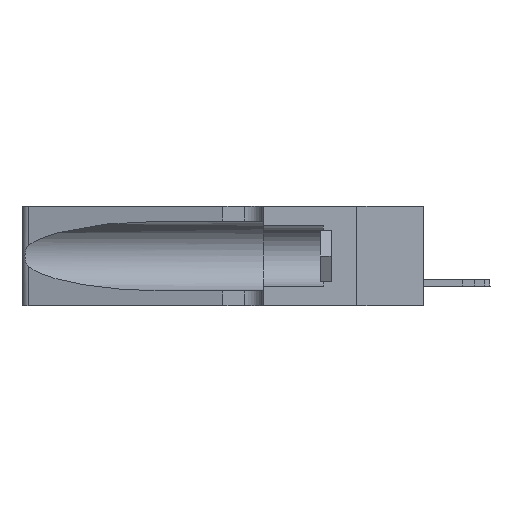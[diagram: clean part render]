
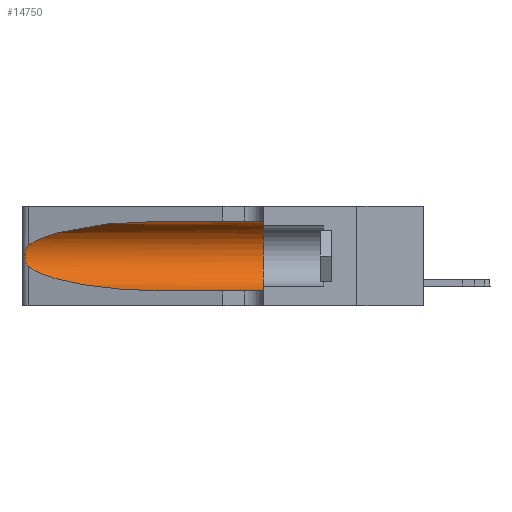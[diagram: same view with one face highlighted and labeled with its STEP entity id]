
A CAD part, left-side view. The second image highlights one B-rep face of the part: STEP entity #14750.
In plain terms, the highlighted cylindrical face has radius 3.308 mm (diameter 6.617 mm), a partial arc.
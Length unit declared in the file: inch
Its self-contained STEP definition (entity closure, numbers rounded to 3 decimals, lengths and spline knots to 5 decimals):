
#248 = CARTESIAN_POINT ( 'NONE',  ( 0.25854, 1.2359, 0.20912 ) ) ;
#848 = CARTESIAN_POINT ( 'NONE',  ( 0.25487, 1.22718, 0.14631 ) ) ;
#2346 = AXIS2_PLACEMENT_3D ( 'NONE', #15928, #9743, #16616 ) ;
#2508 = CARTESIAN_POINT ( 'NONE',  ( 0.1305, 0.35, 0.05475 ) ) ;
#2638 = DIRECTION ( 'NONE',  ( 0., 0., 1. ) ) ;
#3244 = VERTEX_POINT ( 'NONE', #22983 ) ;
#3895 = VERTEX_POINT ( 'NONE', #26742 ) ;
#4047 = EDGE_CURVE ( 'NONE', #18157, #18648, #27140, .T. ) ;
#4755 = ORIENTED_EDGE ( 'NONE', *, *, #14588, .T. ) ;
#4892 = CARTESIAN_POINT ( 'NONE',  ( 0.25487, 1.22718, 0.14631 ) ) ;
#5075 = CARTESIAN_POINT ( 'NONE',  ( 0.26075, 1.23896, 0.19203 ) ) ;
#5078 = DIRECTION ( 'NONE',  ( 0., -1., 0. ) ) ;
#5647 = VECTOR ( 'NONE', #5078, 39.37008 ) ;
#6132 = CARTESIAN_POINT ( 'NONE',  ( 0.25487, 1.22718, 0.22369 ) ) ;
#6234 = CARTESIAN_POINT ( 'NONE',  ( 0.25555, 1.22994, 0.2215 ) ) ;
#7052 = CARTESIAN_POINT ( 'NONE',  ( 0.1305, 0.72297, 0.31525 ) ) ;
#7231 = CARTESIAN_POINT ( 'NONE',  ( 0.26018, 1.23835, 0.19895 ) ) ;
#7365 = ORIENTED_EDGE ( 'NONE', *, *, #4047, .F. ) ;
#7531 = CARTESIAN_POINT ( 'NONE',  ( 0.25856, 1.23593, 0.16098 ) ) ;
#7639 = EDGE_CURVE ( 'NONE', #11296, #3895, #25047, .T. ) ;
#7738 = EDGE_CURVE ( 'NONE', #3895, #3244, #27250, .T. ) ;
#7966 = CYLINDRICAL_SURFACE ( 'NONE', #2346, 0.13025 ) ;
#8201 = CARTESIAN_POINT ( 'NONE',  ( 0.1305, 1.61858, 0.05475 ) ) ;
#8306 = DIRECTION ( 'NONE',  ( 0., -1., 0. ) ) ;
#9164 = LINE ( 'NONE', #11592, #5647 ) ;
#9306 = CARTESIAN_POINT ( 'NONE',  ( 0.18966, 0.96281, 0.31525 ) ) ;
#9743 = DIRECTION ( 'NONE',  ( 0., -1., 0. ) ) ;
#10112 =( BOUNDED_CURVE ( )  B_SPLINE_CURVE ( 3, ( #4892, #11691, #27488, #16175 ),
 .UNSPECIFIED., .F., .F. ) 
 B_SPLINE_CURVE_WITH_KNOTS ( ( 4, 4 ),
 ( 3.44316, 4.71239 ),
 .UNSPECIFIED. ) 
 CURVE ( )  GEOMETRIC_REPRESENTATION_ITEM ( )  RATIONAL_B_SPLINE_CURVE ( ( 1., 0.87, 0.87, 1. ) ) 
 REPRESENTATION_ITEM ( '' )  );
#11251 = EDGE_LOOP ( 'NONE', ( #20474, #21062, #4755, #28572, #7365, #18052 ) ) ;
#11296 = VERTEX_POINT ( 'NONE', #13615 ) ;
#11592 = CARTESIAN_POINT ( 'NONE',  ( 0.1305, 1.61858, 0.31525 ) ) ;
#11691 = CARTESIAN_POINT ( 'NONE',  ( 0.2373, 1.15595, 0.08982 ) ) ;
#12273 = CARTESIAN_POINT ( 'NONE',  ( 0.25639, 1.23186, 0.15144 ) ) ;
#13034 = EDGE_CURVE ( 'NONE', #16992, #18648, #18766, .T. ) ;
#13615 = CARTESIAN_POINT ( 'NONE',  ( 0.1305, 0.72297, 0.31525 ) ) ;
#13805 = CARTESIAN_POINT ( 'NONE',  ( 0.26075, 1.23896, 0.178 ) ) ;
#13905 = CARTESIAN_POINT ( 'NONE',  ( 0.26017, 1.23833, 0.17102 ) ) ;
#14387 = CARTESIAN_POINT ( 'NONE',  ( 0.1305, 0.72297, 0.05475 ) ) ;
#14588 = EDGE_CURVE ( 'NONE', #3244, #16992, #10112, .T. ) ;
#14750 = ADVANCED_FACE ( 'NONE', ( #16508 ), #7966, .F. ) ;
#15928 = CARTESIAN_POINT ( 'NONE',  ( 0.1305, 1.61858, 0.185 ) ) ;
#16175 = CARTESIAN_POINT ( 'NONE',  ( 0.1305, 0.72297, 0.05475 ) ) ;
#16508 = FACE_OUTER_BOUND ( 'NONE', #11251, .T. ) ;
#16616 = DIRECTION ( 'NONE',  ( 0., 0., -1. ) ) ;
#16992 = VERTEX_POINT ( 'NONE', #14387 ) ;
#18052 = ORIENTED_EDGE ( 'NONE', *, *, #28957, .F. ) ;
#18157 = VERTEX_POINT ( 'NONE', #25216 ) ;
#18260 = CARTESIAN_POINT ( 'NONE',  ( 0.25787, 1.23484, 0.2124 ) ) ;
#18648 = VERTEX_POINT ( 'NONE', #2508 ) ;
#18766 = LINE ( 'NONE', #8201, #25119 ) ;
#20474 = ORIENTED_EDGE ( 'NONE', *, *, #7639, .T. ) ;
#20752 = CARTESIAN_POINT ( 'NONE',  ( 0.25487, 1.22718, 0.22369 ) ) ;
#20764 = CARTESIAN_POINT ( 'NONE',  ( 0.1305, 0.35, 0.185 ) ) ;
#20847 = CARTESIAN_POINT ( 'NONE',  ( 0.25639, 1.23184, 0.21858 ) ) ;
#21062 = ORIENTED_EDGE ( 'NONE', *, *, #7738, .T. ) ;
#22983 = CARTESIAN_POINT ( 'NONE',  ( 0.25487, 1.22718, 0.14631 ) ) ;
#23315 = CARTESIAN_POINT ( 'NONE',  ( 0.25555, 1.22993, 0.14849 ) ) ;
#24937 = DIRECTION ( 'NONE',  ( 0., 1., 0. ) ) ;
#25047 =( BOUNDED_CURVE ( )  B_SPLINE_CURVE ( 3, ( #7052, #9306, #25386, #20752 ),
 .UNSPECIFIED., .F., .F. ) 
 B_SPLINE_CURVE_WITH_KNOTS ( ( 4, 4 ),
 ( 1.5708, 2.84003 ),
 .UNSPECIFIED. ) 
 CURVE ( )  GEOMETRIC_REPRESENTATION_ITEM ( )  RATIONAL_B_SPLINE_CURVE ( ( 1., 0.87, 0.87, 1. ) ) 
 REPRESENTATION_ITEM ( '' )  );
#25119 = VECTOR ( 'NONE', #8306, 39.37008 ) ;
#25216 = CARTESIAN_POINT ( 'NONE',  ( 0.1305, 0.35, 0.31525 ) ) ;
#25386 = CARTESIAN_POINT ( 'NONE',  ( 0.2373, 1.15595, 0.28018 ) ) ;
#26742 = CARTESIAN_POINT ( 'NONE',  ( 0.25487, 1.22718, 0.22369 ) ) ;
#27140 = CIRCLE ( 'NONE', #28516, 0.13025 ) ;
#27250 = B_SPLINE_CURVE_WITH_KNOTS ( 'NONE', 3,
 ( #6132, #6234, #20847, #18260, #248, #7231, #5075, #13805, #13905, #7531, #27993, #12273, #23315, #848 ),
 .UNSPECIFIED., .F., .F.,
 ( 4, 2, 2, 2, 2, 2, 4 ),
 ( 0., 0.00027, 0.00053, 0.00107, 0.0016, 0.00187, 0.00214 ),
 .UNSPECIFIED. ) ;
#27488 = CARTESIAN_POINT ( 'NONE',  ( 0.18966, 0.96281, 0.05475 ) ) ;
#27993 = CARTESIAN_POINT ( 'NONE',  ( 0.25789, 1.23486, 0.15765 ) ) ;
#28516 = AXIS2_PLACEMENT_3D ( 'NONE', #20764, #24937, #2638 ) ;
#28572 = ORIENTED_EDGE ( 'NONE', *, *, #13034, .T. ) ;
#28957 = EDGE_CURVE ( 'NONE', #11296, #18157, #9164, .T. ) ;
